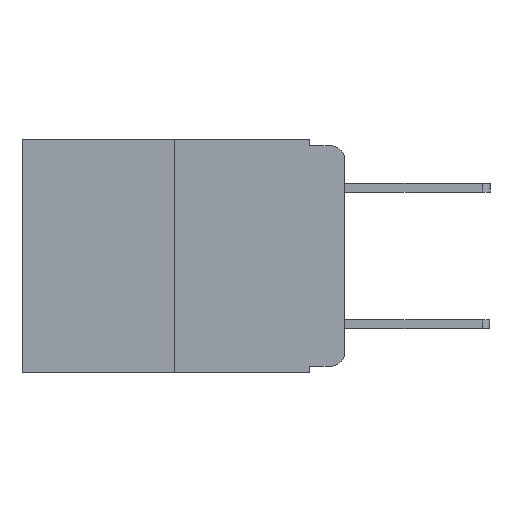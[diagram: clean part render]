
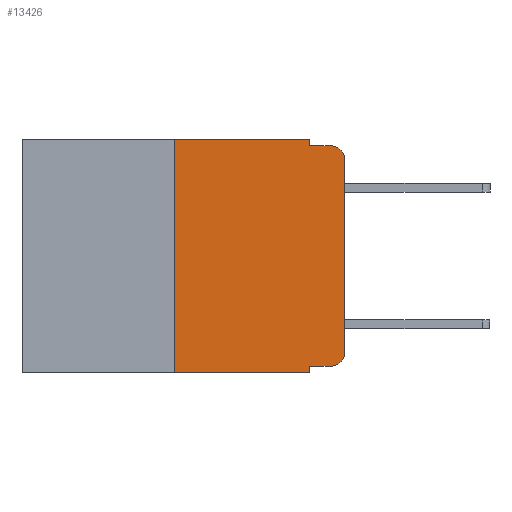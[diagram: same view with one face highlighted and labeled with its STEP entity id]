
A CAD part, left-side view. The second image highlights one B-rep face of the part: STEP entity #13426.
In plain terms, the highlighted planar face has unit normal (-1, 0, 0).
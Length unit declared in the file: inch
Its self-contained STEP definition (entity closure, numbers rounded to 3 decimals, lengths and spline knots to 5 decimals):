
#20 = LINE ( 'NONE', #4777, #17089 ) ;
#104 = DIRECTION ( 'NONE',  ( 0., -1., 0. ) ) ;
#148 = VECTOR ( 'NONE', #8330, 39.37008 ) ;
#153 = CARTESIAN_POINT ( 'NONE',  ( 0., 0.473, 0. ) ) ;
#231 = ORIENTED_EDGE ( 'NONE', *, *, #15998, .F. ) ;
#248 = ORIENTED_EDGE ( 'NONE', *, *, #1251, .T. ) ;
#304 = ORIENTED_EDGE ( 'NONE', *, *, #16819, .F. ) ;
#314 = CARTESIAN_POINT ( 'NONE',  ( 0., 0.02, -0.01 ) ) ;
#323 = EDGE_CURVE ( 'NONE', #3136, #4349, #7972, .T. ) ;
#353 = EDGE_CURVE ( 'NONE', #9092, #3136, #14371, .T. ) ;
#484 = CARTESIAN_POINT ( 'NONE',  ( 0., 0.25, -0.343 ) ) ;
#775 = ORIENTED_EDGE ( 'NONE', *, *, #1282, .T. ) ;
#796 = ORIENTED_EDGE ( 'NONE', *, *, #3358, .T. ) ;
#1140 = EDGE_CURVE ( 'NONE', #15038, #16692, #9212, .T. ) ;
#1251 = EDGE_CURVE ( 'NONE', #16229, #7574, #6146, .T. ) ;
#1282 = EDGE_CURVE ( 'NONE', #2507, #7412, #9405, .T. ) ;
#1501 = CARTESIAN_POINT ( 'NONE',  ( 0., 0.02, -0.03 ) ) ;
#1741 = DIRECTION ( 'NONE',  ( 1., 0., 0. ) ) ;
#2044 = DIRECTION ( 'NONE',  ( 0., 0., -1. ) ) ;
#2100 = DIRECTION ( 'NONE',  ( -1., 0., 0. ) ) ;
#2344 = DIRECTION ( 'NONE',  ( 0., -1., 0. ) ) ;
#2445 = LINE ( 'NONE', #6077, #16131 ) ;
#2507 = VERTEX_POINT ( 'NONE', #7232 ) ;
#3136 = VERTEX_POINT ( 'NONE', #13181 ) ;
#3358 = EDGE_CURVE ( 'NONE', #7412, #9092, #17416, .T. ) ;
#4037 = CARTESIAN_POINT ( 'NONE',  ( 0., 0.473, -0.343 ) ) ;
#4349 = VERTEX_POINT ( 'NONE', #314 ) ;
#4578 = CARTESIAN_POINT ( 'NONE',  ( 0., 0., 0. ) ) ;
#4777 = CARTESIAN_POINT ( 'NONE',  ( 0., 0.051, -0.01 ) ) ;
#5204 = CARTESIAN_POINT ( 'NONE',  ( 0., 0.051, -0.333 ) ) ;
#5270 = VECTOR ( 'NONE', #13328, 39.37008 ) ;
#5500 = VECTOR ( 'NONE', #2344, 39.37008 ) ;
#6066 = AXIS2_PLACEMENT_3D ( 'NONE', #1501, #16992, #15252 ) ;
#6077 = CARTESIAN_POINT ( 'NONE',  ( 0., 0.25, 0. ) ) ;
#6146 = LINE ( 'NONE', #4037, #12829 ) ;
#6184 = DIRECTION ( 'NONE',  ( 0., -1., 0. ) ) ;
#7232 = CARTESIAN_POINT ( 'NONE',  ( 0., 0.051, -0.333 ) ) ;
#7412 = VERTEX_POINT ( 'NONE', #14729 ) ;
#7504 = VECTOR ( 'NONE', #17308, 39.37008 ) ;
#7574 = VERTEX_POINT ( 'NONE', #16265 ) ;
#7669 = CARTESIAN_POINT ( 'NONE',  ( 0., 0.051, 0. ) ) ;
#7860 = EDGE_LOOP ( 'NONE', ( #8673, #8789, #10108, #12325, #13293, #231, #248, #304, #775, #796 ) ) ;
#7972 = CIRCLE ( 'NONE', #6066, 0.02 ) ;
#8330 = DIRECTION ( 'NONE',  ( 0., 0., -1. ) ) ;
#8673 = ORIENTED_EDGE ( 'NONE', *, *, #353, .T. ) ;
#8789 = ORIENTED_EDGE ( 'NONE', *, *, #323, .T. ) ;
#9092 = VERTEX_POINT ( 'NONE', #14383 ) ;
#9212 = LINE ( 'NONE', #10338, #5500 ) ;
#9336 = VECTOR ( 'NONE', #10614, 39.37008 ) ;
#9405 = LINE ( 'NONE', #5204, #5270 ) ;
#10044 = CARTESIAN_POINT ( 'NONE',  ( 0., 0.051, -0.01 ) ) ;
#10108 = ORIENTED_EDGE ( 'NONE', *, *, #14430, .F. ) ;
#10262 = DIRECTION ( 'NONE',  ( 0., 0., 1. ) ) ;
#10338 = CARTESIAN_POINT ( 'NONE',  ( 0., 0.473, 0. ) ) ;
#10614 = DIRECTION ( 'NONE',  ( 0., 0., -1. ) ) ;
#10979 = VERTEX_POINT ( 'NONE', #10044 ) ;
#11559 = DIRECTION ( 'NONE',  ( 0., 0., -1. ) ) ;
#12325 = ORIENTED_EDGE ( 'NONE', *, *, #15221, .F. ) ;
#12651 = CARTESIAN_POINT ( 'NONE',  ( 0., 0.25, 0. ) ) ;
#12760 = LINE ( 'NONE', #7669, #9336 ) ;
#12829 = VECTOR ( 'NONE', #104, 39.37008 ) ;
#13156 = CARTESIAN_POINT ( 'NONE',  ( 0., 0.051, 0. ) ) ;
#13181 = CARTESIAN_POINT ( 'NONE',  ( 0., 0., -0.03 ) ) ;
#13240 = AXIS2_PLACEMENT_3D ( 'NONE', #153, #1741, #11559 ) ;
#13293 = ORIENTED_EDGE ( 'NONE', *, *, #1140, .F. ) ;
#13328 = DIRECTION ( 'NONE',  ( 0., -1., 0. ) ) ;
#13426 = ADVANCED_FACE ( 'NONE', ( #15630 ), #16348, .F. ) ;
#14371 = LINE ( 'NONE', #4578, #7504 ) ;
#14383 = CARTESIAN_POINT ( 'NONE',  ( 0., 0., -0.313 ) ) ;
#14404 = LINE ( 'NONE', #15802, #148 ) ;
#14430 = EDGE_CURVE ( 'NONE', #10979, #4349, #20, .T. ) ;
#14631 = AXIS2_PLACEMENT_3D ( 'NONE', #14822, #2100, #2044 ) ;
#14729 = CARTESIAN_POINT ( 'NONE',  ( 0., 0.02, -0.333 ) ) ;
#14822 = CARTESIAN_POINT ( 'NONE',  ( 0., 0.02, -0.313 ) ) ;
#15038 = VERTEX_POINT ( 'NONE', #12651 ) ;
#15221 = EDGE_CURVE ( 'NONE', #16692, #10979, #12760, .T. ) ;
#15252 = DIRECTION ( 'NONE',  ( 0., 0., -1. ) ) ;
#15630 = FACE_OUTER_BOUND ( 'NONE', #7860, .T. ) ;
#15802 = CARTESIAN_POINT ( 'NONE',  ( 0., 0.051, 0. ) ) ;
#15998 = EDGE_CURVE ( 'NONE', #16229, #15038, #2445, .T. ) ;
#16131 = VECTOR ( 'NONE', #10262, 39.37008 ) ;
#16229 = VERTEX_POINT ( 'NONE', #484 ) ;
#16265 = CARTESIAN_POINT ( 'NONE',  ( 0., 0.051, -0.343 ) ) ;
#16348 = PLANE ( 'NONE',  #13240 ) ;
#16692 = VERTEX_POINT ( 'NONE', #13156 ) ;
#16819 = EDGE_CURVE ( 'NONE', #2507, #7574, #14404, .T. ) ;
#16992 = DIRECTION ( 'NONE',  ( -1., 0., 0. ) ) ;
#17089 = VECTOR ( 'NONE', #6184, 39.37008 ) ;
#17308 = DIRECTION ( 'NONE',  ( 0., 0., 1. ) ) ;
#17416 = CIRCLE ( 'NONE', #14631, 0.02 ) ;
